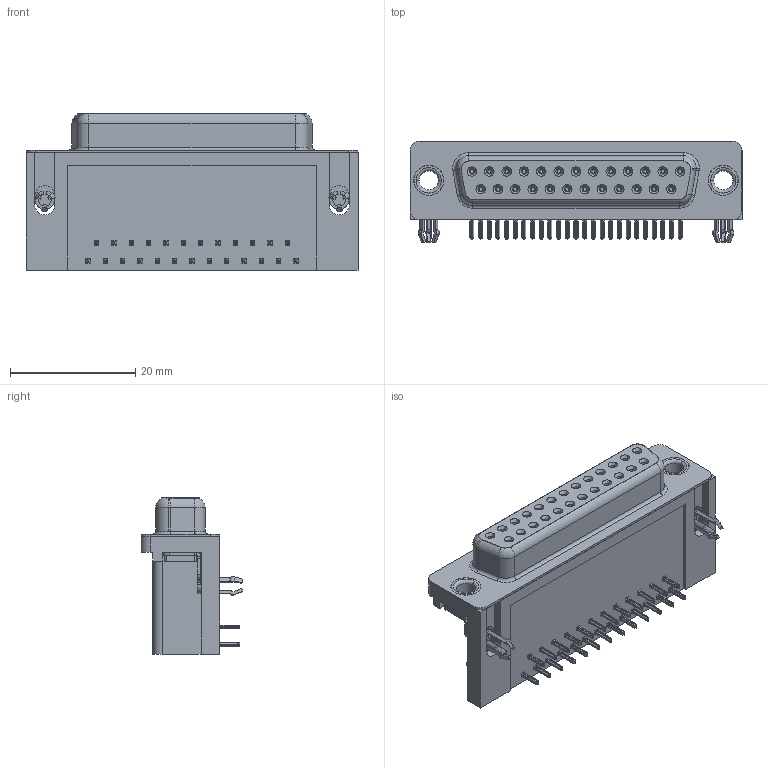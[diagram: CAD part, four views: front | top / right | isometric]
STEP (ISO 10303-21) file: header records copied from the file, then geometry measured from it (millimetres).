
FILE_DESCRIPTION (( 'STEP AP203' ), '1' );
FILE_NAME ('626-025-362-040.STEP', '2018-11-07T03:16:08', ( '' ), ( '' ), 'SwSTEP 2.0', 'SolidWorks 2016', '' );
FILE_SCHEMA (( 'CONFIG_CONTROL_DESIGN' ));
Length unit declared in the file: millimetre
Products named in the file (7): 626 3 Prong Board Lock; 626 Thru Hole Rivet; 626-025-362-040; 626 Housing_25 Socket; 626 Shell_25 Socket; 626 Contact Bottom; 626 Contact Top
Assembly tree (31 placements, depth 2):
  626-025-362-040
    626 Housing_25 Socket
    626 Shell_25 Socket
    626 Contact Bottom  x12
    626 Contact Top  x13
    626 3 Prong Board Lock  x2
    626 Thru Hole Rivet  x2
Bounding box: 53.04 x 16.25 x 24.96 mm (x, y, z)
Volume: 10666.6 mm3; surface area: 11402.4 mm2
Topology: 31 solids, 31 shells, 3914 faces, 10300 edges, 6468 vertices
Faces by surface type: plane 1760, cylinder 908, bspline 852, cone 336, torus 58
Entity records: 30414 total; most frequent: CARTESIAN_POINT 8154, ORIENTED_EDGE 4408, DIRECTION 4144, EDGE_CURVE 2204, LINE 1430, VECTOR 1430, VERTEX_POINT 1410, AXIS2_PLACEMENT_3D 1357
